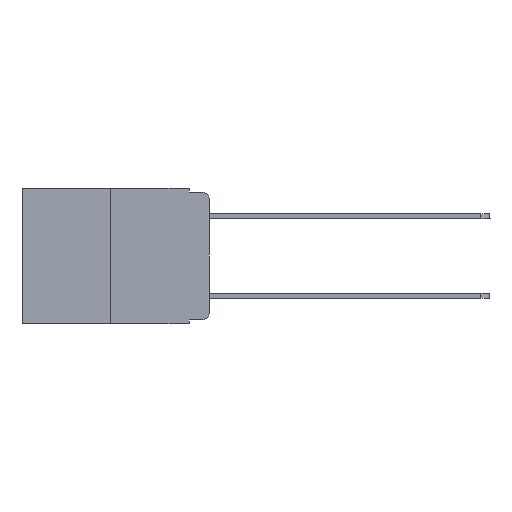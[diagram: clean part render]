
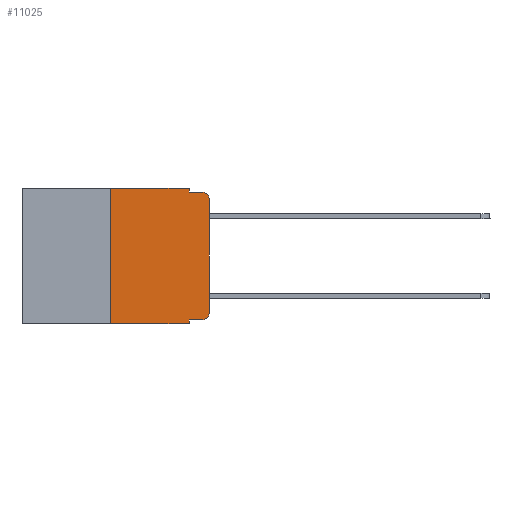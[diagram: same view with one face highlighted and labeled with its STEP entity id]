
A CAD part, left-side view. The second image highlights one B-rep face of the part: STEP entity #11025.
In plain terms, the highlighted planar face has unit normal (-1, 0, 0).
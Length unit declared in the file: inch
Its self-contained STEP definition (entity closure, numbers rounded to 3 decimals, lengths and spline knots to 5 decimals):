
#469 = CARTESIAN_POINT ( 'NONE',  ( 0., 0.25, 0. ) ) ;
#580 = VERTEX_POINT ( 'NONE', #6438 ) ;
#1532 = PLANE ( 'NONE',  #2155 ) ;
#2139 = VERTEX_POINT ( 'NONE', #10655 ) ;
#2155 = AXIS2_PLACEMENT_3D ( 'NONE', #9401, #12991, #13076 ) ;
#2353 = ORIENTED_EDGE ( 'NONE', *, *, #17265, .T. ) ;
#2767 = CARTESIAN_POINT ( 'NONE',  ( 0., 0., 0. ) ) ;
#2975 = CARTESIAN_POINT ( 'NONE',  ( 0., 0.02, -0.01 ) ) ;
#3507 = VECTOR ( 'NONE', #22005, 39.37008 ) ;
#3834 = CARTESIAN_POINT ( 'NONE',  ( 0., 0.051, -0.333 ) ) ;
#4346 = EDGE_CURVE ( 'NONE', #19155, #7765, #6581, .T. ) ;
#5129 = LINE ( 'NONE', #12591, #7781 ) ;
#5172 = CARTESIAN_POINT ( 'NONE',  ( 0., 0.02, -0.333 ) ) ;
#5255 = LINE ( 'NONE', #469, #15876 ) ;
#5308 = ORIENTED_EDGE ( 'NONE', *, *, #14120, .T. ) ;
#5879 = AXIS2_PLACEMENT_3D ( 'NONE', #19522, #19690, #10247 ) ;
#6438 = CARTESIAN_POINT ( 'NONE',  ( 0., 0., -0.313 ) ) ;
#6581 = LINE ( 'NONE', #10600, #11581 ) ;
#7032 = EDGE_CURVE ( 'NONE', #22282, #13043, #15900, .T. ) ;
#7101 = AXIS2_PLACEMENT_3D ( 'NONE', #13106, #22448, #20737 ) ;
#7528 = EDGE_CURVE ( 'NONE', #19155, #22282, #5255, .T. ) ;
#7602 = EDGE_CURVE ( 'NONE', #2139, #21188, #19693, .T. ) ;
#7765 = VERTEX_POINT ( 'NONE', #22052 ) ;
#7781 = VECTOR ( 'NONE', #14086, 39.37008 ) ;
#8840 = EDGE_CURVE ( 'NONE', #13648, #7765, #21649, .T. ) ;
#9401 = CARTESIAN_POINT ( 'NONE',  ( 0., 0.473, 0. ) ) ;
#9909 = ORIENTED_EDGE ( 'NONE', *, *, #20559, .T. ) ;
#10085 = VECTOR ( 'NONE', #24249, 39.37008 ) ;
#10247 = DIRECTION ( 'NONE',  ( 0., 0., -1. ) ) ;
#10282 = VECTOR ( 'NONE', #21404, 39.37008 ) ;
#10600 = CARTESIAN_POINT ( 'NONE',  ( 0., 0.473, -0.343 ) ) ;
#10655 = CARTESIAN_POINT ( 'NONE',  ( 0., 0.051, -0.01 ) ) ;
#10947 = ORIENTED_EDGE ( 'NONE', *, *, #7528, .F. ) ;
#10951 = VERTEX_POINT ( 'NONE', #5172 ) ;
#11025 = ADVANCED_FACE ( 'NONE', ( #13955 ), #1532, .F. ) ;
#11581 = VECTOR ( 'NONE', #12323, 39.37008 ) ;
#11611 = ORIENTED_EDGE ( 'NONE', *, *, #4346, .T. ) ;
#11647 = CARTESIAN_POINT ( 'NONE',  ( 0., 0.25, -0.343 ) ) ;
#12260 = EDGE_CURVE ( 'NONE', #13043, #2139, #23269, .T. ) ;
#12323 = DIRECTION ( 'NONE',  ( 0., -1., 0. ) ) ;
#12591 = CARTESIAN_POINT ( 'NONE',  ( 0., 0.051, -0.333 ) ) ;
#12991 = DIRECTION ( 'NONE',  ( 1., 0., 0. ) ) ;
#13043 = VERTEX_POINT ( 'NONE', #23160 ) ;
#13076 = DIRECTION ( 'NONE',  ( 0., 0., -1. ) ) ;
#13106 = CARTESIAN_POINT ( 'NONE',  ( 0., 0.02, -0.03 ) ) ;
#13618 = DIRECTION ( 'NONE',  ( 0., 0., 1. ) ) ;
#13648 = VERTEX_POINT ( 'NONE', #3834 ) ;
#13955 = FACE_OUTER_BOUND ( 'NONE', #18344, .T. ) ;
#14086 = DIRECTION ( 'NONE',  ( 0., -1., 0. ) ) ;
#14112 = CARTESIAN_POINT ( 'NONE',  ( 0., 0.051, 0. ) ) ;
#14120 = EDGE_CURVE ( 'NONE', #15854, #21188, #20249, .T. ) ;
#14851 = CIRCLE ( 'NONE', #5879, 0.02 ) ;
#15854 = VERTEX_POINT ( 'NONE', #20556 ) ;
#15876 = VECTOR ( 'NONE', #13618, 39.37008 ) ;
#15900 = LINE ( 'NONE', #23801, #3507 ) ;
#16175 = ORIENTED_EDGE ( 'NONE', *, *, #17020, .T. ) ;
#16738 = ORIENTED_EDGE ( 'NONE', *, *, #8840, .F. ) ;
#17020 = EDGE_CURVE ( 'NONE', #10951, #580, #14851, .T. ) ;
#17226 = LINE ( 'NONE', #2767, #20438 ) ;
#17265 = EDGE_CURVE ( 'NONE', #13648, #10951, #5129, .T. ) ;
#17832 = DIRECTION ( 'NONE',  ( 0., 0., 1. ) ) ;
#17867 = ORIENTED_EDGE ( 'NONE', *, *, #7602, .F. ) ;
#18344 = EDGE_LOOP ( 'NONE', ( #9909, #5308, #17867, #18600, #24180, #10947, #11611, #16738, #2353, #16175 ) ) ;
#18600 = ORIENTED_EDGE ( 'NONE', *, *, #12260, .F. ) ;
#19155 = VERTEX_POINT ( 'NONE', #11647 ) ;
#19420 = CARTESIAN_POINT ( 'NONE',  ( 0., 0.25, 0. ) ) ;
#19522 = CARTESIAN_POINT ( 'NONE',  ( 0., 0.02, -0.313 ) ) ;
#19690 = DIRECTION ( 'NONE',  ( -1., 0., 0. ) ) ;
#19693 = LINE ( 'NONE', #23369, #10282 ) ;
#20249 = CIRCLE ( 'NONE', #7101, 0.02 ) ;
#20438 = VECTOR ( 'NONE', #17832, 39.37008 ) ;
#20470 = CARTESIAN_POINT ( 'NONE',  ( 0., 0.051, 0. ) ) ;
#20556 = CARTESIAN_POINT ( 'NONE',  ( 0., 0., -0.03 ) ) ;
#20559 = EDGE_CURVE ( 'NONE', #580, #15854, #17226, .T. ) ;
#20737 = DIRECTION ( 'NONE',  ( 0., 0., -1. ) ) ;
#21056 = VECTOR ( 'NONE', #23265, 39.37008 ) ;
#21188 = VERTEX_POINT ( 'NONE', #2975 ) ;
#21404 = DIRECTION ( 'NONE',  ( 0., -1., 0. ) ) ;
#21649 = LINE ( 'NONE', #14112, #21056 ) ;
#22005 = DIRECTION ( 'NONE',  ( 0., -1., 0. ) ) ;
#22052 = CARTESIAN_POINT ( 'NONE',  ( 0., 0.051, -0.343 ) ) ;
#22282 = VERTEX_POINT ( 'NONE', #19420 ) ;
#22448 = DIRECTION ( 'NONE',  ( -1., 0., 0. ) ) ;
#23160 = CARTESIAN_POINT ( 'NONE',  ( 0., 0.051, 0. ) ) ;
#23265 = DIRECTION ( 'NONE',  ( 0., 0., -1. ) ) ;
#23269 = LINE ( 'NONE', #20470, #10085 ) ;
#23369 = CARTESIAN_POINT ( 'NONE',  ( 0., 0.051, -0.01 ) ) ;
#23801 = CARTESIAN_POINT ( 'NONE',  ( 0., 0.473, 0. ) ) ;
#24180 = ORIENTED_EDGE ( 'NONE', *, *, #7032, .F. ) ;
#24249 = DIRECTION ( 'NONE',  ( 0., 0., -1. ) ) ;
